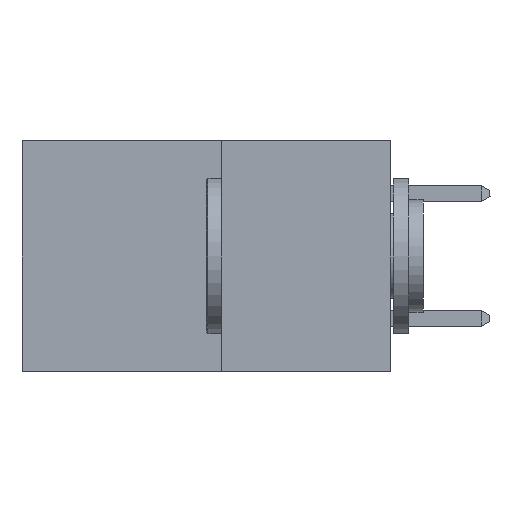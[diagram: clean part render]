
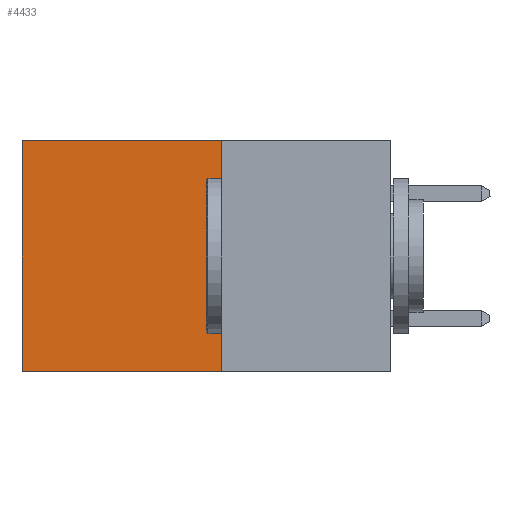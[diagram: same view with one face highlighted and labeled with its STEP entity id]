
A CAD part, left-side view. The second image highlights one B-rep face of the part: STEP entity #4433.
In plain terms, the highlighted planar face has unit normal (-1, 0, 0).
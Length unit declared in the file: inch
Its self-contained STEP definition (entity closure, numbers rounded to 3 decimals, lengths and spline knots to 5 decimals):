
#264 = EDGE_LOOP ( 'NONE', ( #16220, #5641, #17765, #6683 ) ) ;
#3955 = VECTOR ( 'NONE', #16093, 39.37008 ) ;
#4433 = ADVANCED_FACE ( 'NONE', ( #14320 ), #27265, .F. ) ;
#4520 = EDGE_CURVE ( 'NONE', #26718, #26686, #7330, .T. ) ;
#5641 = ORIENTED_EDGE ( 'NONE', *, *, #5989, .F. ) ;
#5989 = EDGE_CURVE ( 'NONE', #25464, #26686, #26538, .T. ) ;
#6683 = ORIENTED_EDGE ( 'NONE', *, *, #25067, .T. ) ;
#7330 = LINE ( 'NONE', #17064, #12331 ) ;
#8830 = CARTESIAN_POINT ( 'NONE',  ( 0.277, 0.27, -0.37 ) ) ;
#11369 = VERTEX_POINT ( 'NONE', #26388 ) ;
#12278 = LINE ( 'NONE', #26690, #3955 ) ;
#12331 = VECTOR ( 'NONE', #13369, 39.37008 ) ;
#12986 = DIRECTION ( 'NONE',  ( 0., 1., 0. ) ) ;
#13196 = CARTESIAN_POINT ( 'NONE',  ( 0.277, 0.27, -0.37 ) ) ;
#13369 = DIRECTION ( 'NONE',  ( 0., 0., -1. ) ) ;
#14320 = FACE_OUTER_BOUND ( 'NONE', #264, .T. ) ;
#14750 = CARTESIAN_POINT ( 'NONE',  ( 0.277, 0.59, 0. ) ) ;
#15799 = EDGE_CURVE ( 'NONE', #11369, #25464, #12278, .T. ) ;
#16093 = DIRECTION ( 'NONE',  ( 0., 0., -1. ) ) ;
#16220 = ORIENTED_EDGE ( 'NONE', *, *, #4520, .T. ) ;
#16721 = CARTESIAN_POINT ( 'NONE',  ( 0.277, 0.59, -0.37 ) ) ;
#17064 = CARTESIAN_POINT ( 'NONE',  ( 0.277, 0.59, -0.37 ) ) ;
#17365 = LINE ( 'NONE', #24097, #21064 ) ;
#17765 = ORIENTED_EDGE ( 'NONE', *, *, #15799, .F. ) ;
#21064 = VECTOR ( 'NONE', #24179, 39.37008 ) ;
#22096 = AXIS2_PLACEMENT_3D ( 'NONE', #27261, #26824, #26935 ) ;
#24097 = CARTESIAN_POINT ( 'NONE',  ( 0.277, 0.27, 0. ) ) ;
#24179 = DIRECTION ( 'NONE',  ( 0., 1., 0. ) ) ;
#25067 = EDGE_CURVE ( 'NONE', #11369, #26718, #17365, .T. ) ;
#25464 = VERTEX_POINT ( 'NONE', #8830 ) ;
#25872 = VECTOR ( 'NONE', #12986, 39.37008 ) ;
#26388 = CARTESIAN_POINT ( 'NONE',  ( 0.277, 0.27, 0. ) ) ;
#26538 = LINE ( 'NONE', #13196, #25872 ) ;
#26686 = VERTEX_POINT ( 'NONE', #16721 ) ;
#26690 = CARTESIAN_POINT ( 'NONE',  ( 0.277, 0.27, -0.37 ) ) ;
#26718 = VERTEX_POINT ( 'NONE', #14750 ) ;
#26824 = DIRECTION ( 'NONE',  ( 1., 0., 0. ) ) ;
#26935 = DIRECTION ( 'NONE',  ( 0., 0., -1. ) ) ;
#27261 = CARTESIAN_POINT ( 'NONE',  ( 0.277, 0.27, -0.37 ) ) ;
#27265 = PLANE ( 'NONE',  #22096 ) ;
